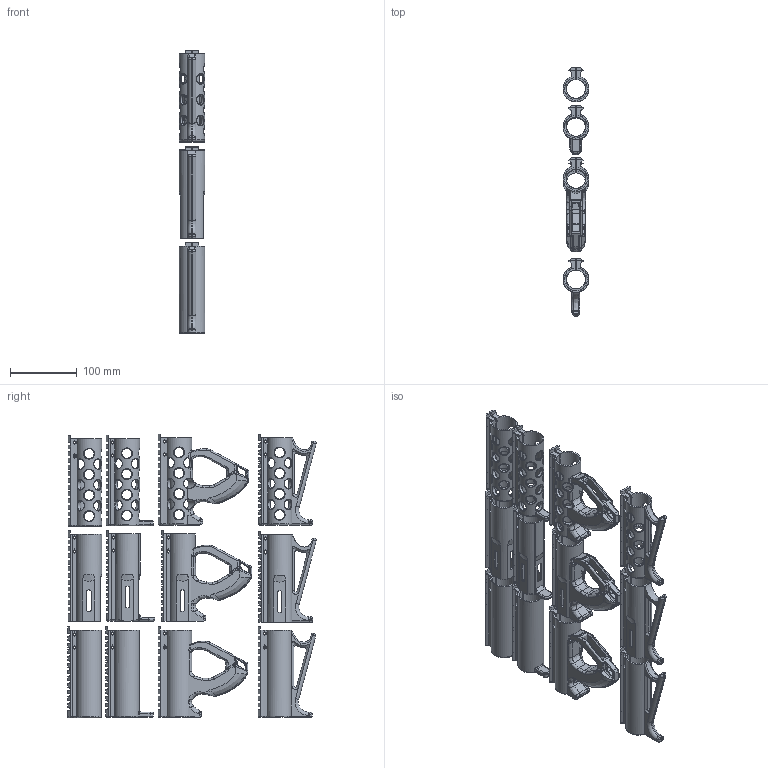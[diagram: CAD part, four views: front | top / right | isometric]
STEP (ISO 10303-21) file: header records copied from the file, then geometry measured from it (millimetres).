
FILE_DESCRIPTION(/* description */ (''),/* implementation_level */ '2;1');
FILE_NAME(/* name */ 'Handguards v21_step.stp',/* time_stamp */ '2022-09-04T10:34:20-04:00',/* author */ (''),/* organization */ (''),/* preprocessor_version */ 'ST-DEVELOPER v16.7',/* originating_system */ 'SIEMENS PLM Software NX 1899',/* authorisation */ '');
FILE_SCHEMA (('AUTOMOTIVE_DESIGN { 1 0 10303 214 3 1 1 1 }'));
Length unit declared in the file: millimetre
Products named in the file (1): tyle2B58769Bow4m
Bounding box: 38.49 x 370.92 x 423.58 mm (x, y, z)
Volume: 1104067.1 mm3; surface area: 490600.6 mm2
Topology: 12 solids, 12 shells, 2999 faces, 8434 edges, 5399 vertices
Faces by surface type: plane 1571, cylinder 541, bspline 502, extrusion 228, cone 102, torus 53, sphere 2
Full cylindrical faces by diameter (mm): 3.5 x48, 5.7 x24, 15 x88, 28.5 x12
Entity records: 140636 total; most frequent: CARTESIAN_POINT 67399, ORIENTED_EDGE 16804, DIRECTION 12611, EDGE_CURVE 8402, VERTEX_POINT 5399, VECTOR 5361, LINE 5133, AXIS2_PLACEMENT_3D 3625
